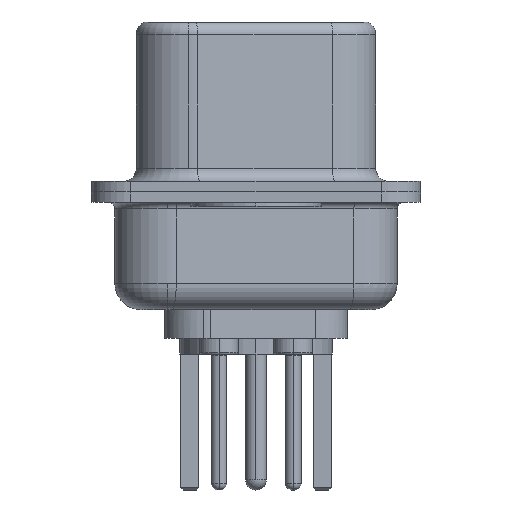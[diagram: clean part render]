
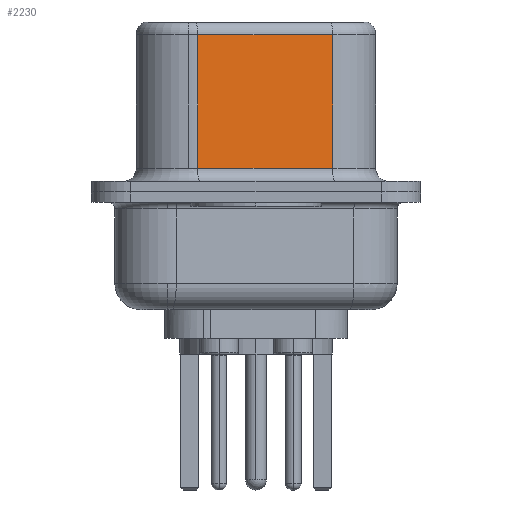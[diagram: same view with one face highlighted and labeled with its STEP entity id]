
A CAD part, left-side view. The second image highlights one B-rep face of the part: STEP entity #2230.
In plain terms, the highlighted planar face has unit normal (-0.985, -0.174, 0).
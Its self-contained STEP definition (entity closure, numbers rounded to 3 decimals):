
#80 = CARTESIAN_POINT ( 'NONE',  ( 4.565, -2.927, 6.52 ) ) ;
#706 = EDGE_CURVE ( 'NONE', #1334, #6600, #4108, .T. ) ;
#1201 = FACE_OUTER_BOUND ( 'NONE', #13931, .T. ) ;
#1325 = EDGE_CURVE ( 'NONE', #8705, #6836, #16947, .T. ) ;
#1334 = VERTEX_POINT ( 'NONE', #15464 ) ;
#2230 = ADVANCED_FACE ( 'NONE', ( #1201 ), #15626, .F. ) ;
#2884 = DIRECTION ( 'NONE',  ( 0., 0., -1. ) ) ;
#4027 = DIRECTION ( 'NONE',  ( -0.174, 0.985, 0. ) ) ;
#4108 = LINE ( 'NONE', #9504, #15011 ) ;
#4234 = ORIENTED_EDGE ( 'NONE', *, *, #1325, .T. ) ;
#4245 = ORIENTED_EDGE ( 'NONE', *, *, #706, .T. ) ;
#5408 = DIRECTION ( 'NONE',  ( -0.174, 0.985, 0. ) ) ;
#5711 = CARTESIAN_POINT ( 'NONE',  ( 4.565, -2.927, 0.9 ) ) ;
#6029 = CARTESIAN_POINT ( 'NONE',  ( 4.565, -2.927, 0.9 ) ) ;
#6163 = ORIENTED_EDGE ( 'NONE', *, *, #9588, .T. ) ;
#6574 = CARTESIAN_POINT ( 'NONE',  ( 4.565, -2.927, 6.52 ) ) ;
#6600 = VERTEX_POINT ( 'NONE', #7452 ) ;
#6836 = VERTEX_POINT ( 'NONE', #6029 ) ;
#6848 = LINE ( 'NONE', #9787, #13753 ) ;
#7452 = CARTESIAN_POINT ( 'NONE',  ( 3.655, 2.233, 6.02 ) ) ;
#8381 = DIRECTION ( 'NONE',  ( 0., 0., -1. ) ) ;
#8669 = LINE ( 'NONE', #80, #15563 ) ;
#8705 = VERTEX_POINT ( 'NONE', #17379 ) ;
#9504 = CARTESIAN_POINT ( 'NONE',  ( 4.565, -2.927, 6.02 ) ) ;
#9588 = EDGE_CURVE ( 'NONE', #6600, #8705, #6848, .T. ) ;
#9787 = CARTESIAN_POINT ( 'NONE',  ( 3.655, 2.233, 6.52 ) ) ;
#12700 = DIRECTION ( 'NONE',  ( 0.985, 0.174, 0. ) ) ;
#12747 = EDGE_CURVE ( 'NONE', #1334, #6836, #8669, .T. ) ;
#13303 = VECTOR ( 'NONE', #14716, 1000. ) ;
#13753 = VECTOR ( 'NONE', #2884, 1000. ) ;
#13914 = ORIENTED_EDGE ( 'NONE', *, *, #12747, .F. ) ;
#13931 = EDGE_LOOP ( 'NONE', ( #13914, #4245, #6163, #4234 ) ) ;
#14716 = DIRECTION ( 'NONE',  ( 0.174, -0.985, 0. ) ) ;
#15011 = VECTOR ( 'NONE', #5408, 1000. ) ;
#15464 = CARTESIAN_POINT ( 'NONE',  ( 4.565, -2.927, 6.02 ) ) ;
#15563 = VECTOR ( 'NONE', #8381, 1000. ) ;
#15626 = PLANE ( 'NONE',  #16386 ) ;
#16386 = AXIS2_PLACEMENT_3D ( 'NONE', #6574, #12700, #4027 ) ;
#16947 = LINE ( 'NONE', #5711, #13303 ) ;
#17379 = CARTESIAN_POINT ( 'NONE',  ( 3.655, 2.233, 0.9 ) ) ;
